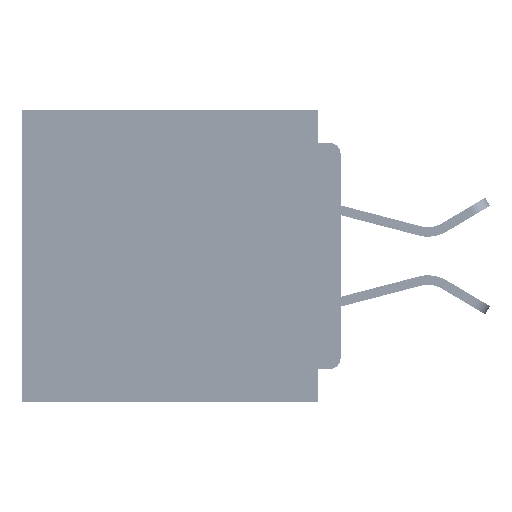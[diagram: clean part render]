
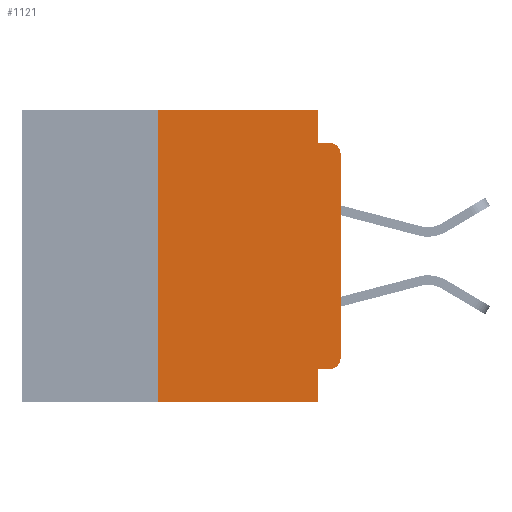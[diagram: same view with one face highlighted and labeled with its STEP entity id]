
A CAD part, left-side view. The second image highlights one B-rep face of the part: STEP entity #1121.
In plain terms, the highlighted planar face has unit normal (-1, 0, 0).
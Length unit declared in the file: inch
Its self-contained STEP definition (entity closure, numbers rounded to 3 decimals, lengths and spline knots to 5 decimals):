
#281 = DIRECTION ( 'NONE',  ( 0., 0., 1. ) ) ;
#1121 = ADVANCED_FACE ( 'NONE', ( #18166 ), #41689, .F. ) ;
#1729 = LINE ( 'NONE', #40534, #38662 ) ;
#2008 = DIRECTION ( 'NONE',  ( 0., -1., 0. ) ) ;
#3521 = VERTEX_POINT ( 'NONE', #23926 ) ;
#3916 = CARTESIAN_POINT ( 'NONE',  ( 0., 0.015, -0.06 ) ) ;
#4408 = DIRECTION ( 'NONE',  ( 0., -1., 0. ) ) ;
#6295 = CARTESIAN_POINT ( 'NONE',  ( 0., 0.25, 0. ) ) ;
#6983 = VECTOR ( 'NONE', #50722, 39.37008 ) ;
#7488 = LINE ( 'NONE', #38064, #41265 ) ;
#8822 = DIRECTION ( 'NONE',  ( 0., 0., -1. ) ) ;
#9090 = CIRCLE ( 'NONE', #59310, 0.015 ) ;
#12029 = CARTESIAN_POINT ( 'NONE',  ( 0., 0.031, 0. ) ) ;
#12556 = CARTESIAN_POINT ( 'NONE',  ( 0., 0.031, -0.045 ) ) ;
#14011 = CARTESIAN_POINT ( 'NONE',  ( 0., 0.031, -0.4 ) ) ;
#15466 = VERTEX_POINT ( 'NONE', #25090 ) ;
#15562 = ORIENTED_EDGE ( 'NONE', *, *, #21112, .F. ) ;
#16890 = VERTEX_POINT ( 'NONE', #12556 ) ;
#17042 = CARTESIAN_POINT ( 'NONE',  ( 0., 0.015, -0.34 ) ) ;
#18166 = FACE_OUTER_BOUND ( 'NONE', #18543, .T. ) ;
#18543 = EDGE_LOOP ( 'NONE', ( #46548, #45172, #55506, #62003, #29075, #29883, #55366, #61048, #15562, #54049 ) ) ;
#18686 = EDGE_CURVE ( 'NONE', #51908, #61641, #9090, .T. ) ;
#19595 = LINE ( 'NONE', #12029, #32384 ) ;
#21112 = EDGE_CURVE ( 'NONE', #33969, #15466, #21232, .T. ) ;
#21232 = LINE ( 'NONE', #36299, #6983 ) ;
#21800 = DIRECTION ( 'NONE',  ( 0., 0., -1. ) ) ;
#22301 = CARTESIAN_POINT ( 'NONE',  ( 0., 0.015, -0.355 ) ) ;
#23830 = EDGE_CURVE ( 'NONE', #31668, #50252, #7488, .T. ) ;
#23926 = CARTESIAN_POINT ( 'NONE',  ( 0., 0.031, -0.4 ) ) ;
#25090 = CARTESIAN_POINT ( 'NONE',  ( 0., 0.031, -0.355 ) ) ;
#28951 = DIRECTION ( 'NONE',  ( 0., 0., -1. ) ) ;
#29075 = ORIENTED_EDGE ( 'NONE', *, *, #23830, .F. ) ;
#29445 = VERTEX_POINT ( 'NONE', #41639 ) ;
#29883 = ORIENTED_EDGE ( 'NONE', *, *, #53379, .F. ) ;
#29922 = DIRECTION ( 'NONE',  ( 1., 0., 0. ) ) ;
#31668 = VERTEX_POINT ( 'NONE', #6295 ) ;
#32384 = VECTOR ( 'NONE', #45602, 39.37008 ) ;
#33489 = EDGE_CURVE ( 'NONE', #15466, #3521, #39072, .T. ) ;
#33533 = LINE ( 'NONE', #50217, #54420 ) ;
#33969 = VERTEX_POINT ( 'NONE', #22301 ) ;
#34523 = EDGE_CURVE ( 'NONE', #33969, #29445, #59721, .T. ) ;
#36046 = AXIS2_PLACEMENT_3D ( 'NONE', #50897, #29922, #28951 ) ;
#36299 = CARTESIAN_POINT ( 'NONE',  ( 0., 0., -0.355 ) ) ;
#36710 = EDGE_CURVE ( 'NONE', #16890, #61641, #1729, .T. ) ;
#37597 = DIRECTION ( 'NONE',  ( -1., 0., 0. ) ) ;
#37682 = VECTOR ( 'NONE', #281, 39.37008 ) ;
#38064 = CARTESIAN_POINT ( 'NONE',  ( 0., 0.437, 0. ) ) ;
#38662 = VECTOR ( 'NONE', #2008, 39.37008 ) ;
#39072 = LINE ( 'NONE', #14011, #54729 ) ;
#39079 = EDGE_CURVE ( 'NONE', #29445, #51908, #50372, .T. ) ;
#39469 = CARTESIAN_POINT ( 'NONE',  ( 0., 0.437, -0.4 ) ) ;
#39816 = LINE ( 'NONE', #39469, #51040 ) ;
#40041 = EDGE_CURVE ( 'NONE', #50252, #16890, #19595, .T. ) ;
#40534 = CARTESIAN_POINT ( 'NONE',  ( 0., 0., -0.045 ) ) ;
#40817 = DIRECTION ( 'NONE',  ( 0., 0., 1. ) ) ;
#41265 = VECTOR ( 'NONE', #4408, 39.37008 ) ;
#41639 = CARTESIAN_POINT ( 'NONE',  ( 0., 0., -0.34 ) ) ;
#41689 = PLANE ( 'NONE',  #36046 ) ;
#44289 = DIRECTION ( 'NONE',  ( 0., -1., 0. ) ) ;
#44500 = CARTESIAN_POINT ( 'NONE',  ( 0., 0.25, -0.4 ) ) ;
#45172 = ORIENTED_EDGE ( 'NONE', *, *, #18686, .T. ) ;
#45602 = DIRECTION ( 'NONE',  ( 0., 0., -1. ) ) ;
#46548 = ORIENTED_EDGE ( 'NONE', *, *, #39079, .T. ) ;
#46988 = CARTESIAN_POINT ( 'NONE',  ( 0., 0.015, -0.045 ) ) ;
#47563 = DIRECTION ( 'NONE',  ( 0., 0., -1. ) ) ;
#47682 = CARTESIAN_POINT ( 'NONE',  ( 0., 0.031, 0. ) ) ;
#48210 = CARTESIAN_POINT ( 'NONE',  ( 0., 0., 0. ) ) ;
#50217 = CARTESIAN_POINT ( 'NONE',  ( 0., 0.25, -0.4 ) ) ;
#50252 = VERTEX_POINT ( 'NONE', #47682 ) ;
#50372 = LINE ( 'NONE', #48210, #37682 ) ;
#50405 = EDGE_CURVE ( 'NONE', #55790, #3521, #39816, .T. ) ;
#50546 = DIRECTION ( 'NONE',  ( -1., 0., 0. ) ) ;
#50722 = DIRECTION ( 'NONE',  ( 0., 1., 0. ) ) ;
#50897 = CARTESIAN_POINT ( 'NONE',  ( 0., 0.437, 0. ) ) ;
#51040 = VECTOR ( 'NONE', #44289, 39.37008 ) ;
#51908 = VERTEX_POINT ( 'NONE', #56371 ) ;
#53379 = EDGE_CURVE ( 'NONE', #55790, #31668, #33533, .T. ) ;
#54049 = ORIENTED_EDGE ( 'NONE', *, *, #34523, .T. ) ;
#54420 = VECTOR ( 'NONE', #40817, 39.37008 ) ;
#54729 = VECTOR ( 'NONE', #47563, 39.37008 ) ;
#55366 = ORIENTED_EDGE ( 'NONE', *, *, #50405, .T. ) ;
#55506 = ORIENTED_EDGE ( 'NONE', *, *, #36710, .F. ) ;
#55790 = VERTEX_POINT ( 'NONE', #44500 ) ;
#56371 = CARTESIAN_POINT ( 'NONE',  ( 0., 0., -0.06 ) ) ;
#59310 = AXIS2_PLACEMENT_3D ( 'NONE', #3916, #37597, #8822 ) ;
#59721 = CIRCLE ( 'NONE', #61429, 0.015 ) ;
#61048 = ORIENTED_EDGE ( 'NONE', *, *, #33489, .F. ) ;
#61429 = AXIS2_PLACEMENT_3D ( 'NONE', #17042, #50546, #21800 ) ;
#61641 = VERTEX_POINT ( 'NONE', #46988 ) ;
#62003 = ORIENTED_EDGE ( 'NONE', *, *, #40041, .F. ) ;
